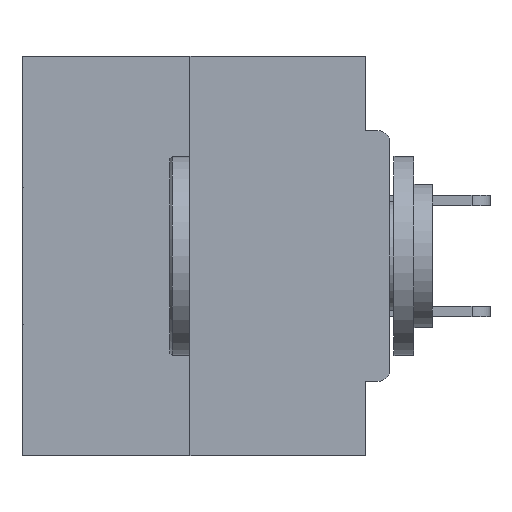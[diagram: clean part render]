
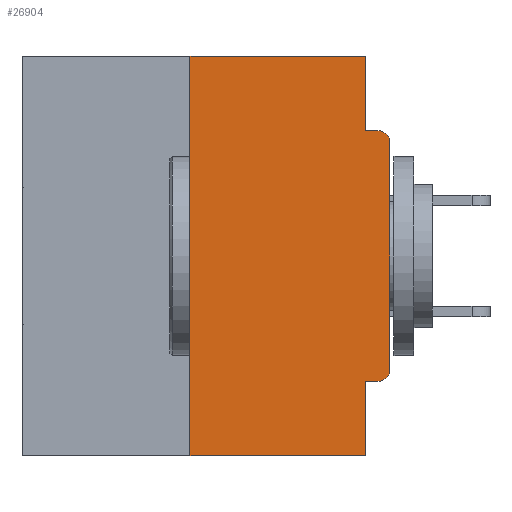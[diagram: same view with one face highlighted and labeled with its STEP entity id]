
A CAD part, left-side view. The second image highlights one B-rep face of the part: STEP entity #26904.
In plain terms, the highlighted planar face has unit normal (-1, 0, 0).
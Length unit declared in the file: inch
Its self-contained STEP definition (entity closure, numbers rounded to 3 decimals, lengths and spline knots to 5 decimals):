
#123 = DIRECTION ( 'NONE',  ( 0., 0., 1. ) ) ;
#366 = AXIS2_PLACEMENT_3D ( 'NONE', #16590, #28647, #31478 ) ;
#471 = CARTESIAN_POINT ( 'NONE',  ( 0., 0.25, 0. ) ) ;
#833 = CARTESIAN_POINT ( 'NONE',  ( 0., 0.031, -0.4065 ) ) ;
#1745 = LINE ( 'NONE', #5717, #38211 ) ;
#1967 = ORIENTED_EDGE ( 'NONE', *, *, #17885, .T. ) ;
#2504 = LINE ( 'NONE', #32728, #17795 ) ;
#2649 = LINE ( 'NONE', #38927, #20818 ) ;
#3980 = VERTEX_POINT ( 'NONE', #471 ) ;
#4850 = EDGE_CURVE ( 'NONE', #13291, #10615, #2649, .T. ) ;
#4912 = DIRECTION ( 'NONE',  ( 0., 0., -1. ) ) ;
#5513 = CARTESIAN_POINT ( 'NONE',  ( 0., 0.031, 0. ) ) ;
#5696 = CARTESIAN_POINT ( 'NONE',  ( 0., 0.46, 0. ) ) ;
#5717 = CARTESIAN_POINT ( 'NONE',  ( 0., 0., 0. ) ) ;
#6039 = ORIENTED_EDGE ( 'NONE', *, *, #36473, .F. ) ;
#6239 = VECTOR ( 'NONE', #26921, 39.37008 ) ;
#6340 = EDGE_CURVE ( 'NONE', #19523, #3980, #11599, .T. ) ;
#6511 = VERTEX_POINT ( 'NONE', #36276 ) ;
#7688 = CARTESIAN_POINT ( 'NONE',  ( 0., 0., -0.0935 ) ) ;
#7974 = FACE_OUTER_BOUND ( 'NONE', #12108, .T. ) ;
#8079 = VECTOR ( 'NONE', #27496, 39.37008 ) ;
#8209 = CARTESIAN_POINT ( 'NONE',  ( 0., 0., -0.1085 ) ) ;
#8620 = CIRCLE ( 'NONE', #11773, 0.015 ) ;
#8653 = ORIENTED_EDGE ( 'NONE', *, *, #6340, .F. ) ;
#10111 = VERTEX_POINT ( 'NONE', #14562 ) ;
#10615 = VERTEX_POINT ( 'NONE', #833 ) ;
#11125 = VECTOR ( 'NONE', #123, 39.37008 ) ;
#11599 = LINE ( 'NONE', #36845, #11125 ) ;
#11773 = AXIS2_PLACEMENT_3D ( 'NONE', #20397, #17194, #4912 ) ;
#12108 = EDGE_LOOP ( 'NONE', ( #6039, #8653, #20487, #27042, #21402, #26513, #1967, #30923, #35657, #37767 ) ) ;
#12423 = LINE ( 'NONE', #24404, #8079 ) ;
#12597 = EDGE_CURVE ( 'NONE', #36934, #23841, #20182, .T. ) ;
#13224 = EDGE_CURVE ( 'NONE', #13291, #37638, #8620, .T. ) ;
#13291 = VERTEX_POINT ( 'NONE', #29645 ) ;
#14562 = CARTESIAN_POINT ( 'NONE',  ( 0., 0.031, 0. ) ) ;
#16159 = VECTOR ( 'NONE', #34954, 39.37008 ) ;
#16175 = CARTESIAN_POINT ( 'NONE',  ( 0., 0.46, 0. ) ) ;
#16590 = CARTESIAN_POINT ( 'NONE',  ( 0., 0.015, -0.1085 ) ) ;
#17194 = DIRECTION ( 'NONE',  ( -1., 0., 0. ) ) ;
#17710 = LINE ( 'NONE', #7688, #6239 ) ;
#17750 = DIRECTION ( 'NONE',  ( 1., 0., 0. ) ) ;
#17795 = VECTOR ( 'NONE', #35714, 39.37008 ) ;
#17874 = DIRECTION ( 'NONE',  ( 0., 0., -1. ) ) ;
#17885 = EDGE_CURVE ( 'NONE', #37638, #36934, #1745, .T. ) ;
#19523 = VERTEX_POINT ( 'NONE', #35224 ) ;
#19618 = CARTESIAN_POINT ( 'NONE',  ( 0., 0., -0.3915 ) ) ;
#19871 = VERTEX_POINT ( 'NONE', #21888 ) ;
#20182 = CIRCLE ( 'NONE', #366, 0.015 ) ;
#20397 = CARTESIAN_POINT ( 'NONE',  ( 0., 0.015, -0.3915 ) ) ;
#20487 = ORIENTED_EDGE ( 'NONE', *, *, #25872, .T. ) ;
#20818 = VECTOR ( 'NONE', #37646, 39.37008 ) ;
#21224 = DIRECTION ( 'NONE',  ( 0., 0., 1. ) ) ;
#21402 = ORIENTED_EDGE ( 'NONE', *, *, #4850, .F. ) ;
#21888 = CARTESIAN_POINT ( 'NONE',  ( 0., 0.031, -0.0935 ) ) ;
#22377 = AXIS2_PLACEMENT_3D ( 'NONE', #5696, #17750, #17874 ) ;
#22523 = EDGE_CURVE ( 'NONE', #10111, #19871, #26571, .T. ) ;
#23841 = VERTEX_POINT ( 'NONE', #27938 ) ;
#23867 = PLANE ( 'NONE',  #22377 ) ;
#24404 = CARTESIAN_POINT ( 'NONE',  ( 0., 0.46, -0.5 ) ) ;
#25606 = VECTOR ( 'NONE', #36216, 39.37008 ) ;
#25872 = EDGE_CURVE ( 'NONE', #19523, #6511, #12423, .T. ) ;
#26513 = ORIENTED_EDGE ( 'NONE', *, *, #13224, .T. ) ;
#26571 = LINE ( 'NONE', #5513, #25606 ) ;
#26904 = ADVANCED_FACE ( 'NONE', ( #7974 ), #23867, .F. ) ;
#26921 = DIRECTION ( 'NONE',  ( 0., -1., 0. ) ) ;
#27042 = ORIENTED_EDGE ( 'NONE', *, *, #39533, .F. ) ;
#27496 = DIRECTION ( 'NONE',  ( 0., -1., 0. ) ) ;
#27938 = CARTESIAN_POINT ( 'NONE',  ( 0., 0.015, -0.0935 ) ) ;
#28647 = DIRECTION ( 'NONE',  ( -1., 0., 0. ) ) ;
#29645 = CARTESIAN_POINT ( 'NONE',  ( 0., 0.015, -0.4065 ) ) ;
#30923 = ORIENTED_EDGE ( 'NONE', *, *, #12597, .T. ) ;
#30998 = LINE ( 'NONE', #16175, #16159 ) ;
#31478 = DIRECTION ( 'NONE',  ( 0., 0., -1. ) ) ;
#32728 = CARTESIAN_POINT ( 'NONE',  ( 0., 0.031, -0.5 ) ) ;
#34731 = EDGE_CURVE ( 'NONE', #19871, #23841, #17710, .T. ) ;
#34954 = DIRECTION ( 'NONE',  ( 0., -1., 0. ) ) ;
#35224 = CARTESIAN_POINT ( 'NONE',  ( 0., 0.25, -0.5 ) ) ;
#35657 = ORIENTED_EDGE ( 'NONE', *, *, #34731, .F. ) ;
#35714 = DIRECTION ( 'NONE',  ( 0., 0., -1. ) ) ;
#36216 = DIRECTION ( 'NONE',  ( 0., 0., -1. ) ) ;
#36276 = CARTESIAN_POINT ( 'NONE',  ( 0., 0.031, -0.5 ) ) ;
#36473 = EDGE_CURVE ( 'NONE', #3980, #10111, #30998, .T. ) ;
#36845 = CARTESIAN_POINT ( 'NONE',  ( 0., 0.25, 0. ) ) ;
#36934 = VERTEX_POINT ( 'NONE', #8209 ) ;
#37638 = VERTEX_POINT ( 'NONE', #19618 ) ;
#37646 = DIRECTION ( 'NONE',  ( 0., 1., 0. ) ) ;
#37767 = ORIENTED_EDGE ( 'NONE', *, *, #22523, .F. ) ;
#38211 = VECTOR ( 'NONE', #21224, 39.37008 ) ;
#38927 = CARTESIAN_POINT ( 'NONE',  ( 0., 0., -0.4065 ) ) ;
#39533 = EDGE_CURVE ( 'NONE', #10615, #6511, #2504, .T. ) ;
